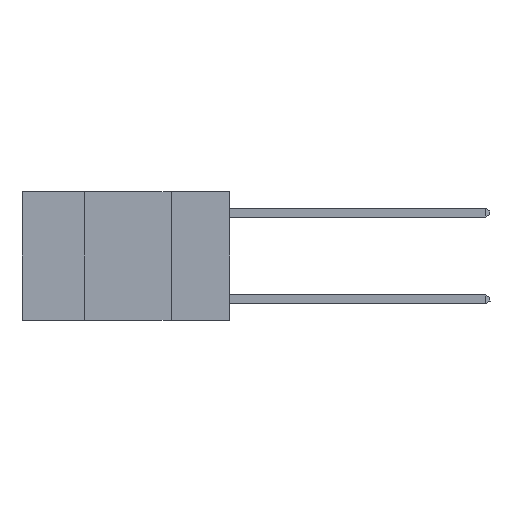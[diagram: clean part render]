
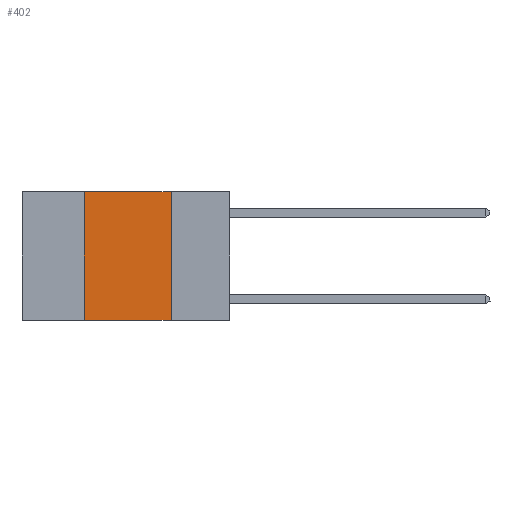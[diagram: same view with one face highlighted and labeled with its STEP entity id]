
A CAD part, left-side view. The second image highlights one B-rep face of the part: STEP entity #402.
In plain terms, the highlighted planar face has unit normal (-1, 0, 0).
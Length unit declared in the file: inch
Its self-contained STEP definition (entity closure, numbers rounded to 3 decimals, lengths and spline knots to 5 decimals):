
#402 = ADVANCED_FACE ( 'NONE', ( #13480 ), #828, .F. ) ;
#556 = VERTEX_POINT ( 'NONE', #10732 ) ;
#828 = PLANE ( 'NONE',  #13620 ) ;
#878 = DIRECTION ( 'NONE',  ( 0., -1., 0. ) ) ;
#891 = EDGE_CURVE ( 'NONE', #6369, #7184, #3747, .T. ) ;
#1333 = DIRECTION ( 'NONE',  ( 0., 0., -1. ) ) ;
#3111 = VECTOR ( 'NONE', #11503, 39.37008 ) ;
#3562 = EDGE_CURVE ( 'NONE', #6369, #12402, #3588, .T. ) ;
#3588 = LINE ( 'NONE', #6343, #11841 ) ;
#3696 = DIRECTION ( 'NONE',  ( 0., 0., 1. ) ) ;
#3747 = LINE ( 'NONE', #8529, #11998 ) ;
#4414 = EDGE_LOOP ( 'NONE', ( #7236, #7187, #13062, #7684 ) ) ;
#5016 = CARTESIAN_POINT ( 'NONE',  ( 0., 0.6, 0. ) ) ;
#5614 = LINE ( 'NONE', #5016, #3111 ) ;
#6343 = CARTESIAN_POINT ( 'NONE',  ( 0., 0.6, -0.37 ) ) ;
#6369 = VERTEX_POINT ( 'NONE', #12931 ) ;
#6618 = CARTESIAN_POINT ( 'NONE',  ( 0., 0.42, 0. ) ) ;
#6801 = CARTESIAN_POINT ( 'NONE',  ( 0., 0.17, 0. ) ) ;
#7184 = VERTEX_POINT ( 'NONE', #6618 ) ;
#7187 = ORIENTED_EDGE ( 'NONE', *, *, #10080, .F. ) ;
#7236 = ORIENTED_EDGE ( 'NONE', *, *, #8130, .F. ) ;
#7684 = ORIENTED_EDGE ( 'NONE', *, *, #3562, .T. ) ;
#7916 = LINE ( 'NONE', #6801, #10427 ) ;
#8130 = EDGE_CURVE ( 'NONE', #556, #12402, #7916, .T. ) ;
#8157 = CARTESIAN_POINT ( 'NONE',  ( 0., 0.17, -0.37 ) ) ;
#8529 = CARTESIAN_POINT ( 'NONE',  ( 0., 0.42, 0. ) ) ;
#9651 = DIRECTION ( 'NONE',  ( 0., 0., -1. ) ) ;
#10080 = EDGE_CURVE ( 'NONE', #7184, #556, #5614, .T. ) ;
#10427 = VECTOR ( 'NONE', #1333, 39.37008 ) ;
#10732 = CARTESIAN_POINT ( 'NONE',  ( 0., 0.17, 0. ) ) ;
#11503 = DIRECTION ( 'NONE',  ( 0., -1., 0. ) ) ;
#11841 = VECTOR ( 'NONE', #878, 39.37008 ) ;
#11998 = VECTOR ( 'NONE', #3696, 39.37008 ) ;
#12159 = CARTESIAN_POINT ( 'NONE',  ( 0., 0.6, 0. ) ) ;
#12402 = VERTEX_POINT ( 'NONE', #8157 ) ;
#12931 = CARTESIAN_POINT ( 'NONE',  ( 0., 0.42, -0.37 ) ) ;
#13062 = ORIENTED_EDGE ( 'NONE', *, *, #891, .F. ) ;
#13480 = FACE_OUTER_BOUND ( 'NONE', #4414, .T. ) ;
#13620 = AXIS2_PLACEMENT_3D ( 'NONE', #12159, #13801, #9651 ) ;
#13801 = DIRECTION ( 'NONE',  ( 1., 0., 0. ) ) ;
